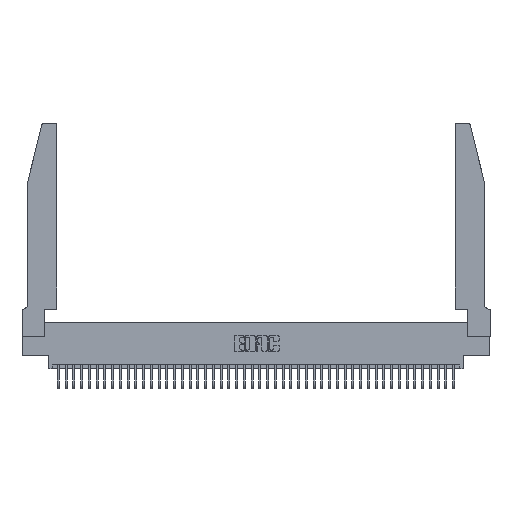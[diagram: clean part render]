
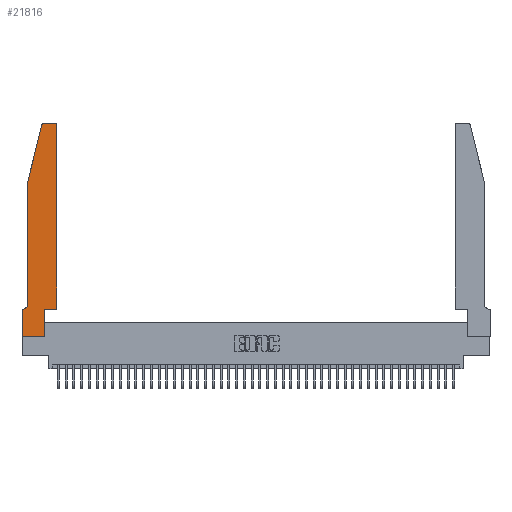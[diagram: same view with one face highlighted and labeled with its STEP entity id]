
A CAD part, top view. The second image highlights one B-rep face of the part: STEP entity #21816.
In plain terms, the highlighted planar face has unit normal (0, 0, 1).
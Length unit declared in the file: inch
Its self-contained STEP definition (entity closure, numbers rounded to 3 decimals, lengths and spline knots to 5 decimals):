
#341 = DIRECTION ( 'NONE',  ( 1., 0., 0. ) ) ;
#404 = DIRECTION ( 'NONE',  ( 1., 0., 0. ) ) ;
#765 = EDGE_CURVE ( 'NONE', #21036, #15131, #13199, .T. ) ;
#888 = AXIS2_PLACEMENT_3D ( 'NONE', #16855, #20163, #341 ) ;
#1480 = VERTEX_POINT ( 'NONE', #39037 ) ;
#2261 = DIRECTION ( 'NONE',  ( 1., 0., 0. ) ) ;
#2882 = CARTESIAN_POINT ( 'NONE',  ( 0.4505, 2.72, 0.37 ) ) ;
#3002 = ORIENTED_EDGE ( 'NONE', *, *, #26096, .T. ) ;
#3107 = DIRECTION ( 'NONE',  ( 1., 0., 0. ) ) ;
#3881 = LINE ( 'NONE', #37654, #19373 ) ;
#4270 = ORIENTED_EDGE ( 'NONE', *, *, #765, .T. ) ;
#5863 = CARTESIAN_POINT ( 'NONE',  ( 0.0055, 0.35, 0.37 ) ) ;
#6136 = CARTESIAN_POINT ( 'NONE',  ( 0., 0., 0.37 ) ) ;
#6418 = LINE ( 'NONE', #9284, #40493 ) ;
#6767 = EDGE_CURVE ( 'NONE', #8934, #31335, #35911, .T. ) ;
#7289 = EDGE_CURVE ( 'NONE', #31609, #13534, #6418, .T. ) ;
#8298 = CARTESIAN_POINT ( 'NONE',  ( 0.2865, 0., 0.37 ) ) ;
#8934 = VERTEX_POINT ( 'NONE', #5863 ) ;
#8973 = VERTEX_POINT ( 'NONE', #6136 ) ;
#9284 = CARTESIAN_POINT ( 'NONE',  ( 0.2865, 0.35, 0.37 ) ) ;
#9441 = EDGE_LOOP ( 'NONE', ( #34945, #23481, #30442, #36494, #41850, #41168, #3002, #40058, #9534, #39839, #40689, #4270 ) ) ;
#9534 = ORIENTED_EDGE ( 'NONE', *, *, #7289, .T. ) ;
#9786 = CARTESIAN_POINT ( 'NONE',  ( 0.0755, 2., 0.37 ) ) ;
#9849 = AXIS2_PLACEMENT_3D ( 'NONE', #18348, #41380, #21644 ) ;
#10212 = CARTESIAN_POINT ( 'NONE',  ( 0.0055, 0.42, 0.37 ) ) ;
#11246 = EDGE_CURVE ( 'NONE', #1480, #8934, #33490, .T. ) ;
#12862 = DIRECTION ( 'NONE',  ( 0., -1., 0. ) ) ;
#13100 = AXIS2_PLACEMENT_3D ( 'NONE', #10212, #33267, #13500 ) ;
#13199 = CIRCLE ( 'NONE', #9849, 0.03 ) ;
#13498 = DIRECTION ( 'NONE',  ( -1., 0., 0. ) ) ;
#13500 = DIRECTION ( 'NONE',  ( -1., 0., 0. ) ) ;
#13534 = VERTEX_POINT ( 'NONE', #14639 ) ;
#13543 = VECTOR ( 'NONE', #2261, 39.37008 ) ;
#14639 = CARTESIAN_POINT ( 'NONE',  ( 0.2865, 0.35, 0.37 ) ) ;
#14941 = EDGE_CURVE ( 'NONE', #13534, #24301, #36681, .T. ) ;
#15131 = VERTEX_POINT ( 'NONE', #17147 ) ;
#16855 = CARTESIAN_POINT ( 'NONE',  ( 0., 0.35, 0.37 ) ) ;
#17147 = CARTESIAN_POINT ( 'NONE',  ( 0.4205, 2.75, 0.37 ) ) ;
#17905 = VERTEX_POINT ( 'NONE', #36234 ) ;
#18348 = CARTESIAN_POINT ( 'NONE',  ( 0.4205, 2.72, 0.37 ) ) ;
#18764 = CARTESIAN_POINT ( 'NONE',  ( 0., 0., 0.37 ) ) ;
#19373 = VECTOR ( 'NONE', #40965, 39.37008 ) ;
#19406 = VECTOR ( 'NONE', #13498, 39.37008 ) ;
#19435 = EDGE_CURVE ( 'NONE', #17905, #42560, #30316, .T. ) ;
#19722 = EDGE_CURVE ( 'NONE', #24301, #21036, #22038, .T. ) ;
#19983 = VECTOR ( 'NONE', #21758, 39.37008 ) ;
#20163 = DIRECTION ( 'NONE',  ( 0., 0., 1. ) ) ;
#20219 = DIRECTION ( 'NONE',  ( 0., 0., 1. ) ) ;
#21036 = VERTEX_POINT ( 'NONE', #2882 ) ;
#21644 = DIRECTION ( 'NONE',  ( 1., 0., 0. ) ) ;
#21718 = VERTEX_POINT ( 'NONE', #9786 ) ;
#21758 = DIRECTION ( 'NONE',  ( 0., 1., 0. ) ) ;
#21816 = ADVANCED_FACE ( 'NONE', ( #36766 ), #36573, .T. ) ;
#22038 = LINE ( 'NONE', #25056, #19983 ) ;
#22187 = VECTOR ( 'NONE', #12862, 39.37008 ) ;
#22875 = CARTESIAN_POINT ( 'NONE',  ( 0.4505, 0.35, 0.37 ) ) ;
#23481 = ORIENTED_EDGE ( 'NONE', *, *, #19435, .T. ) ;
#23841 = LINE ( 'NONE', #37956, #40342 ) ;
#24301 = VERTEX_POINT ( 'NONE', #26132 ) ;
#25056 = CARTESIAN_POINT ( 'NONE',  ( 0.4505, 0.35, 0.37 ) ) ;
#26096 = EDGE_CURVE ( 'NONE', #31335, #8973, #3881, .T. ) ;
#26132 = CARTESIAN_POINT ( 'NONE',  ( 0.4505, 0.35, 0.37 ) ) ;
#28487 = EDGE_CURVE ( 'NONE', #8973, #31609, #32112, .T. ) ;
#29813 = EDGE_CURVE ( 'NONE', #21718, #1480, #39730, .T. ) ;
#29936 = CARTESIAN_POINT ( 'NONE',  ( 0., 0.35, 0.37 ) ) ;
#29973 = VECTOR ( 'NONE', #3107, 39.37008 ) ;
#30316 = CIRCLE ( 'NONE', #36222, 0.03 ) ;
#30442 = ORIENTED_EDGE ( 'NONE', *, *, #37988, .T. ) ;
#31335 = VERTEX_POINT ( 'NONE', #29936 ) ;
#31609 = VERTEX_POINT ( 'NONE', #8298 ) ;
#32112 = LINE ( 'NONE', #18764, #13543 ) ;
#32228 = CARTESIAN_POINT ( 'NONE',  ( 0.2605, 2.75, 0.37 ) ) ;
#32370 = DIRECTION ( 'NONE',  ( -1., 0., 0. ) ) ;
#33267 = DIRECTION ( 'NONE',  ( 0., 0., -1. ) ) ;
#33490 = CIRCLE ( 'NONE', #13100, 0.07 ) ;
#34733 = LINE ( 'NONE', #32228, #40390 ) ;
#34945 = ORIENTED_EDGE ( 'NONE', *, *, #37540, .T. ) ;
#35805 = DIRECTION ( 'NONE',  ( 0., 1., 0. ) ) ;
#35911 = LINE ( 'NONE', #36567, #19406 ) ;
#35985 = CARTESIAN_POINT ( 'NONE',  ( 0.25487, 2.72718, 0.37 ) ) ;
#36222 = AXIS2_PLACEMENT_3D ( 'NONE', #39938, #20219, #404 ) ;
#36234 = CARTESIAN_POINT ( 'NONE',  ( 0.284, 2.75, 0.37 ) ) ;
#36494 = ORIENTED_EDGE ( 'NONE', *, *, #29813, .T. ) ;
#36567 = CARTESIAN_POINT ( 'NONE',  ( 0.0755, 0.35, 0.37 ) ) ;
#36573 = PLANE ( 'NONE',  #888 ) ;
#36681 = LINE ( 'NONE', #22875, #29973 ) ;
#36766 = FACE_OUTER_BOUND ( 'NONE', #9441, .T. ) ;
#37540 = EDGE_CURVE ( 'NONE', #15131, #17905, #34733, .T. ) ;
#37654 = CARTESIAN_POINT ( 'NONE',  ( 0., 0., 0.37 ) ) ;
#37956 = CARTESIAN_POINT ( 'NONE',  ( 0.0755, 2., 0.37 ) ) ;
#37988 = EDGE_CURVE ( 'NONE', #42560, #21718, #23841, .T. ) ;
#39037 = CARTESIAN_POINT ( 'NONE',  ( 0.0755, 0.42, 0.37 ) ) ;
#39730 = LINE ( 'NONE', #42383, #22187 ) ;
#39839 = ORIENTED_EDGE ( 'NONE', *, *, #14941, .T. ) ;
#39938 = CARTESIAN_POINT ( 'NONE',  ( 0.284, 2.72, 0.37 ) ) ;
#40058 = ORIENTED_EDGE ( 'NONE', *, *, #28487, .T. ) ;
#40342 = VECTOR ( 'NONE', #41268, 39.37008 ) ;
#40390 = VECTOR ( 'NONE', #32370, 39.37008 ) ;
#40493 = VECTOR ( 'NONE', #35805, 39.37008 ) ;
#40689 = ORIENTED_EDGE ( 'NONE', *, *, #19722, .T. ) ;
#40965 = DIRECTION ( 'NONE',  ( 0., -1., 0. ) ) ;
#41168 = ORIENTED_EDGE ( 'NONE', *, *, #6767, .T. ) ;
#41268 = DIRECTION ( 'NONE',  ( -0.239, -0.971, 0. ) ) ;
#41380 = DIRECTION ( 'NONE',  ( 0., 0., 1. ) ) ;
#41850 = ORIENTED_EDGE ( 'NONE', *, *, #11246, .T. ) ;
#42383 = CARTESIAN_POINT ( 'NONE',  ( 0.0755, 2., 0.37 ) ) ;
#42560 = VERTEX_POINT ( 'NONE', #35985 ) ;
